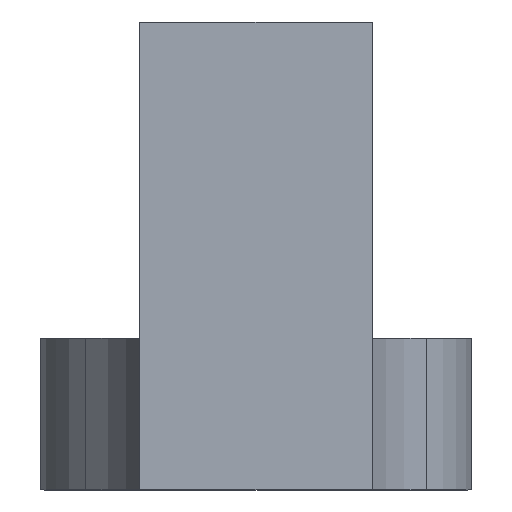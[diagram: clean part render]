
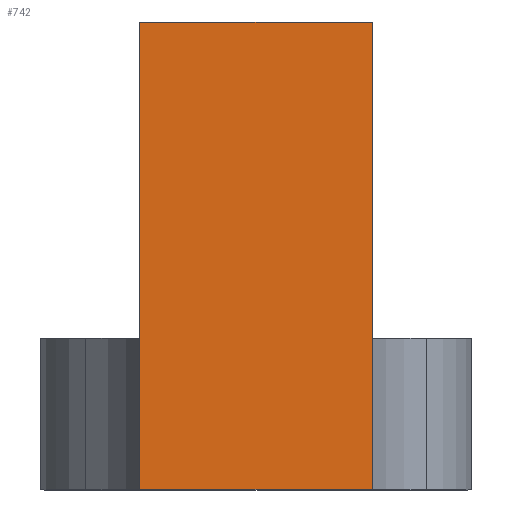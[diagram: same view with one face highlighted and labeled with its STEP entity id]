
A CAD part, top view. The second image highlights one B-rep face of the part: STEP entity #742.
In plain terms, the highlighted planar face has unit normal (0, 0, 1).
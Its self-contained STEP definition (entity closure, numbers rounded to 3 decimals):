
#2 = CARTESIAN_POINT ( 'NONE',  ( 9.5, 20.08, 9. ) ) ;
#5 = EDGE_CURVE ( 'NONE', #260, #444, #364, .T. ) ;
#129 = PLANE ( 'NONE',  #550 ) ;
#131 = VECTOR ( 'NONE', #615, 1000. ) ;
#147 = EDGE_CURVE ( 'NONE', #260, #158, #262, .T. ) ;
#158 = VERTEX_POINT ( 'NONE', #2 ) ;
#215 = CARTESIAN_POINT ( 'NONE',  ( -0.5, 0., 9. ) ) ;
#220 = CARTESIAN_POINT ( 'NONE',  ( -0.5, 6.5, 9. ) ) ;
#221 = CARTESIAN_POINT ( 'NONE',  ( 9.5, 0., 9. ) ) ;
#238 = DIRECTION ( 'NONE',  ( 1., 0., 0. ) ) ;
#249 = EDGE_LOOP ( 'NONE', ( #614, #281, #414, #462 ) ) ;
#260 = VERTEX_POINT ( 'NONE', #485 ) ;
#262 = LINE ( 'NONE', #565, #318 ) ;
#271 = DIRECTION ( 'NONE',  ( 1., 0., 0. ) ) ;
#273 = VECTOR ( 'NONE', #332, 1000. ) ;
#281 = ORIENTED_EDGE ( 'NONE', *, *, #569, .F. ) ;
#283 = LINE ( 'NONE', #381, #131 ) ;
#318 = VECTOR ( 'NONE', #238, 1000. ) ;
#332 = DIRECTION ( 'NONE',  ( 0., -1., 0. ) ) ;
#364 = LINE ( 'NONE', #220, #273 ) ;
#381 = CARTESIAN_POINT ( 'NONE',  ( 9.5, 6.5, 9. ) ) ;
#414 = ORIENTED_EDGE ( 'NONE', *, *, #147, .F. ) ;
#444 = VERTEX_POINT ( 'NONE', #472 ) ;
#462 = ORIENTED_EDGE ( 'NONE', *, *, #5, .T. ) ;
#463 = LINE ( 'NONE', #215, #586 ) ;
#472 = CARTESIAN_POINT ( 'NONE',  ( -0.5, 0., 9. ) ) ;
#485 = CARTESIAN_POINT ( 'NONE',  ( -0.5, 20.08, 9. ) ) ;
#512 = DIRECTION ( 'NONE',  ( 0., 0., -1. ) ) ;
#543 = EDGE_CURVE ( 'NONE', #444, #580, #463, .T. ) ;
#550 = AXIS2_PLACEMENT_3D ( 'NONE', #697, #512, #583 ) ;
#555 = FACE_OUTER_BOUND ( 'NONE', #249, .T. ) ;
#565 = CARTESIAN_POINT ( 'NONE',  ( -0.5, 20.08, 9. ) ) ;
#569 = EDGE_CURVE ( 'NONE', #158, #580, #283, .T. ) ;
#580 = VERTEX_POINT ( 'NONE', #221 ) ;
#583 = DIRECTION ( 'NONE',  ( -1., 0., 0. ) ) ;
#586 = VECTOR ( 'NONE', #271, 1000. ) ;
#614 = ORIENTED_EDGE ( 'NONE', *, *, #543, .T. ) ;
#615 = DIRECTION ( 'NONE',  ( 0., -1., 0. ) ) ;
#697 = CARTESIAN_POINT ( 'NONE',  ( -0.5, 6.5, 9. ) ) ;
#742 = ADVANCED_FACE ( 'NONE', ( #555 ), #129, .F. ) ;
